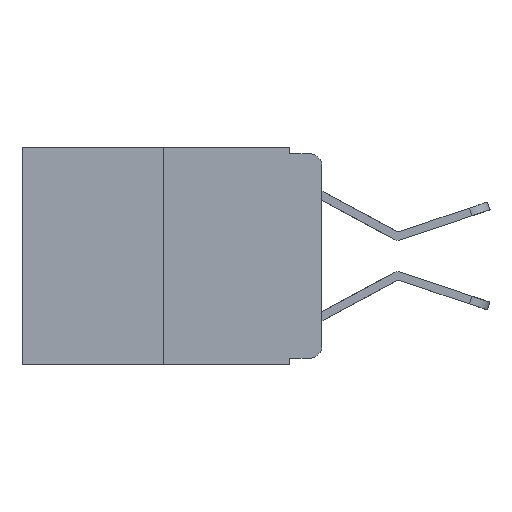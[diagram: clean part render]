
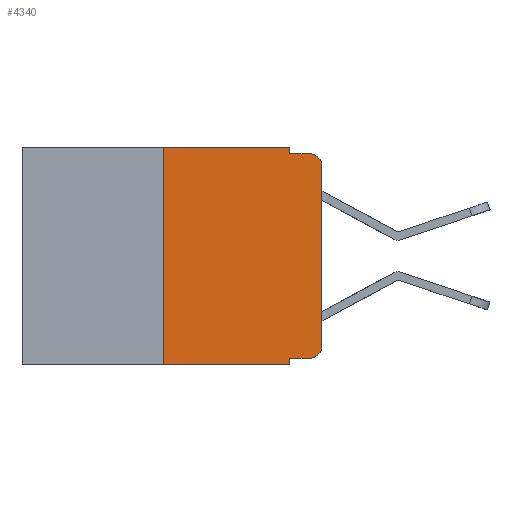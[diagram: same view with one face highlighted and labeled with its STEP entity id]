
A CAD part, left-side view. The second image highlights one B-rep face of the part: STEP entity #4340.
In plain terms, the highlighted planar face has unit normal (-1, 0, 0).
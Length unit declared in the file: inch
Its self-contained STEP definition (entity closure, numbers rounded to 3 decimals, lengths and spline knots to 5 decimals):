
#542 = EDGE_CURVE ( 'NONE', #15038, #9722, #3187, .T. ) ;
#616 = CARTESIAN_POINT ( 'NONE',  ( 0., 0.051, -0.01 ) ) ;
#1210 = CARTESIAN_POINT ( 'NONE',  ( 0., 0.02, -0.313 ) ) ;
#1593 = DIRECTION ( 'NONE',  ( -1., 0., 0. ) ) ;
#1622 = DIRECTION ( 'NONE',  ( 0., 0., -1. ) ) ;
#1662 = ORIENTED_EDGE ( 'NONE', *, *, #2277, .T. ) ;
#1804 = CARTESIAN_POINT ( 'NONE',  ( 0., 0.051, -0.333 ) ) ;
#2084 = DIRECTION ( 'NONE',  ( 0., 0., -1. ) ) ;
#2254 = PLANE ( 'NONE',  #2576 ) ;
#2277 = EDGE_CURVE ( 'NONE', #8962, #17014, #12653, .T. ) ;
#2294 = CARTESIAN_POINT ( 'NONE',  ( 0., 0.473, 0. ) ) ;
#2334 = VERTEX_POINT ( 'NONE', #1804 ) ;
#2410 = FACE_OUTER_BOUND ( 'NONE', #5642, .T. ) ;
#2534 = DIRECTION ( 'NONE',  ( 1., 0., 0. ) ) ;
#2576 = AXIS2_PLACEMENT_3D ( 'NONE', #16459, #2534, #9730 ) ;
#2728 = CARTESIAN_POINT ( 'NONE',  ( 0., 0., 0. ) ) ;
#3014 = CARTESIAN_POINT ( 'NONE',  ( 0., 0.473, -0.343 ) ) ;
#3187 = LINE ( 'NONE', #2294, #17835 ) ;
#3217 = LINE ( 'NONE', #10504, #6491 ) ;
#3545 = DIRECTION ( 'NONE',  ( 0., -1., 0. ) ) ;
#3693 = CARTESIAN_POINT ( 'NONE',  ( 0., 0.02, -0.01 ) ) ;
#4340 = ADVANCED_FACE ( 'NONE', ( #2410 ), #2254, .F. ) ;
#4376 = ORIENTED_EDGE ( 'NONE', *, *, #10693, .F. ) ;
#4835 = ORIENTED_EDGE ( 'NONE', *, *, #16161, .T. ) ;
#4945 = CARTESIAN_POINT ( 'NONE',  ( 0., 0.051, -0.01 ) ) ;
#4989 = VERTEX_POINT ( 'NONE', #7073 ) ;
#5118 = LINE ( 'NONE', #10451, #5540 ) ;
#5143 = EDGE_CURVE ( 'NONE', #2334, #8962, #10488, .T. ) ;
#5540 = VECTOR ( 'NONE', #2084, 39.37008 ) ;
#5642 = EDGE_LOOP ( 'NONE', ( #4835, #9799, #14498, #4376, #10001, #10454, #10217, #16410, #11481, #1662 ) ) ;
#5851 = VECTOR ( 'NONE', #13806, 39.37008 ) ;
#5969 = AXIS2_PLACEMENT_3D ( 'NONE', #1210, #17919, #1622 ) ;
#6040 = EDGE_CURVE ( 'NONE', #2334, #8187, #7004, .T. ) ;
#6491 = VECTOR ( 'NONE', #14888, 39.37008 ) ;
#6795 = VECTOR ( 'NONE', #3545, 39.37008 ) ;
#6797 = CARTESIAN_POINT ( 'NONE',  ( 0., 0.051, -0.333 ) ) ;
#6940 = VERTEX_POINT ( 'NONE', #3693 ) ;
#7004 = LINE ( 'NONE', #11442, #14733 ) ;
#7058 = LINE ( 'NONE', #616, #17140 ) ;
#7073 = CARTESIAN_POINT ( 'NONE',  ( 0., 0., -0.03 ) ) ;
#7219 = VERTEX_POINT ( 'NONE', #4945 ) ;
#7918 = EDGE_CURVE ( 'NONE', #17747, #15038, #3217, .T. ) ;
#8139 = CARTESIAN_POINT ( 'NONE',  ( 0., 0.25, 0. ) ) ;
#8187 = VERTEX_POINT ( 'NONE', #13355 ) ;
#8962 = VERTEX_POINT ( 'NONE', #14319 ) ;
#9132 = CARTESIAN_POINT ( 'NONE',  ( 0., 0.25, -0.343 ) ) ;
#9542 = LINE ( 'NONE', #2728, #5851 ) ;
#9722 = VERTEX_POINT ( 'NONE', #12410 ) ;
#9730 = DIRECTION ( 'NONE',  ( 0., 0., -1. ) ) ;
#9799 = ORIENTED_EDGE ( 'NONE', *, *, #15255, .T. ) ;
#9978 = CARTESIAN_POINT ( 'NONE',  ( 0., 0.02, -0.03 ) ) ;
#10001 = ORIENTED_EDGE ( 'NONE', *, *, #542, .F. ) ;
#10006 = CIRCLE ( 'NONE', #12654, 0.02 ) ;
#10090 = DIRECTION ( 'NONE',  ( 0., 0., -1. ) ) ;
#10217 = ORIENTED_EDGE ( 'NONE', *, *, #16302, .T. ) ;
#10451 = CARTESIAN_POINT ( 'NONE',  ( 0., 0.051, 0. ) ) ;
#10454 = ORIENTED_EDGE ( 'NONE', *, *, #7918, .F. ) ;
#10488 = LINE ( 'NONE', #6797, #6795 ) ;
#10504 = CARTESIAN_POINT ( 'NONE',  ( 0., 0.25, 0. ) ) ;
#10629 = VECTOR ( 'NONE', #14086, 39.37008 ) ;
#10693 = EDGE_CURVE ( 'NONE', #9722, #7219, #5118, .T. ) ;
#11353 = DIRECTION ( 'NONE',  ( 0., 0., -1. ) ) ;
#11442 = CARTESIAN_POINT ( 'NONE',  ( 0., 0.051, 0. ) ) ;
#11481 = ORIENTED_EDGE ( 'NONE', *, *, #5143, .T. ) ;
#11625 = CARTESIAN_POINT ( 'NONE',  ( 0., 0., -0.313 ) ) ;
#12410 = CARTESIAN_POINT ( 'NONE',  ( 0., 0.051, 0. ) ) ;
#12499 = EDGE_CURVE ( 'NONE', #7219, #6940, #7058, .T. ) ;
#12653 = CIRCLE ( 'NONE', #5969, 0.02 ) ;
#12654 = AXIS2_PLACEMENT_3D ( 'NONE', #9978, #1593, #11353 ) ;
#13355 = CARTESIAN_POINT ( 'NONE',  ( 0., 0.051, -0.343 ) ) ;
#13806 = DIRECTION ( 'NONE',  ( 0., 0., 1. ) ) ;
#14086 = DIRECTION ( 'NONE',  ( 0., -1., 0. ) ) ;
#14319 = CARTESIAN_POINT ( 'NONE',  ( 0., 0.02, -0.333 ) ) ;
#14498 = ORIENTED_EDGE ( 'NONE', *, *, #12499, .F. ) ;
#14672 = LINE ( 'NONE', #3014, #10629 ) ;
#14733 = VECTOR ( 'NONE', #10090, 39.37008 ) ;
#14888 = DIRECTION ( 'NONE',  ( 0., 0., 1. ) ) ;
#15038 = VERTEX_POINT ( 'NONE', #8139 ) ;
#15255 = EDGE_CURVE ( 'NONE', #4989, #6940, #10006, .T. ) ;
#15678 = DIRECTION ( 'NONE',  ( 0., -1., 0. ) ) ;
#15871 = DIRECTION ( 'NONE',  ( 0., -1., 0. ) ) ;
#16161 = EDGE_CURVE ( 'NONE', #17014, #4989, #9542, .T. ) ;
#16302 = EDGE_CURVE ( 'NONE', #17747, #8187, #14672, .T. ) ;
#16410 = ORIENTED_EDGE ( 'NONE', *, *, #6040, .F. ) ;
#16459 = CARTESIAN_POINT ( 'NONE',  ( 0., 0.473, 0. ) ) ;
#17014 = VERTEX_POINT ( 'NONE', #11625 ) ;
#17140 = VECTOR ( 'NONE', #15871, 39.37008 ) ;
#17747 = VERTEX_POINT ( 'NONE', #9132 ) ;
#17835 = VECTOR ( 'NONE', #15678, 39.37008 ) ;
#17919 = DIRECTION ( 'NONE',  ( -1., 0., 0. ) ) ;
